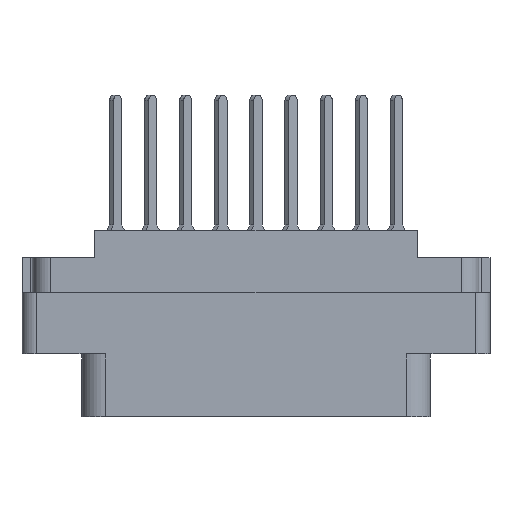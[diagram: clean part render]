
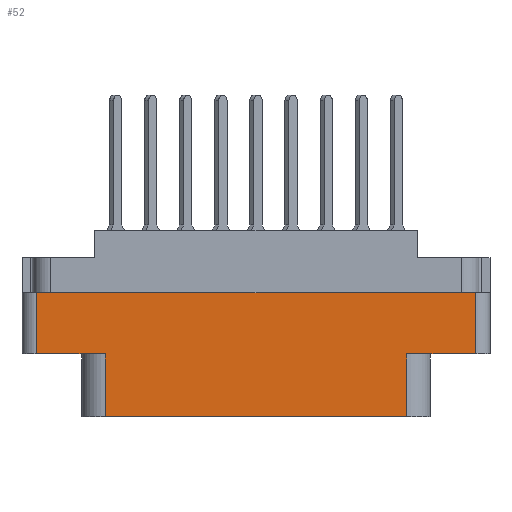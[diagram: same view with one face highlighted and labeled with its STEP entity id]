
A CAD part, front view. The second image highlights one B-rep face of the part: STEP entity #52.
In plain terms, the highlighted planar face has unit normal (0, -1, 0).
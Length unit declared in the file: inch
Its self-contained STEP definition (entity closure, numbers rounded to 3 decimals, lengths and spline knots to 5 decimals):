
#52 = ADVANCED_FACE ( 'NONE', ( #8722 ), #30549, .T. ) ;
#787 = DIRECTION ( 'NONE',  ( 1., 0., 0. ) ) ;
#976 = CARTESIAN_POINT ( 'NONE',  ( 0.644, -0.438, -0.798 ) ) ;
#1190 = DIRECTION ( 'NONE',  ( 1., 0., 0. ) ) ;
#1614 = LINE ( 'NONE', #27000, #14510 ) ;
#1641 = VERTEX_POINT ( 'NONE', #27500 ) ;
#3336 = ORIENTED_EDGE ( 'NONE', *, *, #4127, .F. ) ;
#4081 = CARTESIAN_POINT ( 'NONE',  ( -0.938, -0.438, -0.798 ) ) ;
#4127 = EDGE_CURVE ( 'NONE', #13085, #1641, #29717, .T. ) ;
#4637 = VERTEX_POINT ( 'NONE', #976 ) ;
#5229 = CARTESIAN_POINT ( 'NONE',  ( -1., -0.438, -0.268 ) ) ;
#5317 = EDGE_CURVE ( 'NONE', #13085, #31289, #1614, .T. ) ;
#5384 = DIRECTION ( 'NONE',  ( -1., 0., 0. ) ) ;
#5725 = DIRECTION ( 'NONE',  ( 0., -1., 0. ) ) ;
#6505 = VERTEX_POINT ( 'NONE', #16839 ) ;
#7265 = LINE ( 'NONE', #11999, #16705 ) ;
#7801 = EDGE_LOOP ( 'NONE', ( #8703, #9466, #13724, #3336, #32241, #9646, #20688, #8863 ) ) ;
#7983 = DIRECTION ( 'NONE',  ( 0., 0., -1. ) ) ;
#8046 = DIRECTION ( 'NONE',  ( 1., 0., 0. ) ) ;
#8423 = CARTESIAN_POINT ( 'NONE',  ( -0.938, -0.438, -0.268 ) ) ;
#8432 = CARTESIAN_POINT ( 'NONE',  ( 0., -0.438, -0.529 ) ) ;
#8542 = EDGE_CURVE ( 'NONE', #1641, #4637, #7265, .T. ) ;
#8703 = ORIENTED_EDGE ( 'NONE', *, *, #16300, .T. ) ;
#8722 = FACE_OUTER_BOUND ( 'NONE', #7801, .T. ) ;
#8863 = ORIENTED_EDGE ( 'NONE', *, *, #18747, .T. ) ;
#8896 = CARTESIAN_POINT ( 'NONE',  ( -0.938, -0.438, -0.529 ) ) ;
#9466 = ORIENTED_EDGE ( 'NONE', *, *, #31566, .T. ) ;
#9646 = ORIENTED_EDGE ( 'NONE', *, *, #26502, .F. ) ;
#10174 = LINE ( 'NONE', #5229, #15712 ) ;
#10607 = VERTEX_POINT ( 'NONE', #23777 ) ;
#11999 = CARTESIAN_POINT ( 'NONE',  ( 0.644, -0.438, -0.529 ) ) ;
#12372 = DIRECTION ( 'NONE',  ( 0., 0., 1. ) ) ;
#12681 = CARTESIAN_POINT ( 'NONE',  ( 0.938, -0.438, -0.268 ) ) ;
#13085 = VERTEX_POINT ( 'NONE', #28790 ) ;
#13250 = AXIS2_PLACEMENT_3D ( 'NONE', #13253, #5725, #7983 ) ;
#13253 = CARTESIAN_POINT ( 'NONE',  ( -0.938, -0.438, -0.798 ) ) ;
#13724 = ORIENTED_EDGE ( 'NONE', *, *, #8542, .F. ) ;
#14510 = VECTOR ( 'NONE', #17215, 39.37008 ) ;
#14715 = VECTOR ( 'NONE', #787, 39.37008 ) ;
#15229 = DIRECTION ( 'NONE',  ( 0., 0., -1. ) ) ;
#15712 = VECTOR ( 'NONE', #8046, 39.37008 ) ;
#16188 = EDGE_CURVE ( 'NONE', #23786, #16444, #28349, .T. ) ;
#16300 = EDGE_CURVE ( 'NONE', #6505, #10607, #24042, .T. ) ;
#16444 = VERTEX_POINT ( 'NONE', #8423 ) ;
#16563 = DIRECTION ( 'NONE',  ( 0., 0., -1. ) ) ;
#16705 = VECTOR ( 'NONE', #16563, 39.37008 ) ;
#16839 = CARTESIAN_POINT ( 'NONE',  ( -0.644, -0.438, -0.529 ) ) ;
#17092 = VECTOR ( 'NONE', #1190, 39.37008 ) ;
#17215 = DIRECTION ( 'NONE',  ( 0., 0., 1. ) ) ;
#18747 = EDGE_CURVE ( 'NONE', #23786, #6505, #19066, .T. ) ;
#19066 = LINE ( 'NONE', #8432, #14715 ) ;
#19281 = VECTOR ( 'NONE', #15229, 39.37008 ) ;
#20405 = CARTESIAN_POINT ( 'NONE',  ( 0., -0.438, -0.529 ) ) ;
#20688 = ORIENTED_EDGE ( 'NONE', *, *, #16188, .F. ) ;
#22978 = LINE ( 'NONE', #4081, #17092 ) ;
#23049 = CARTESIAN_POINT ( 'NONE',  ( -0.644, -0.438, -0.529 ) ) ;
#23777 = CARTESIAN_POINT ( 'NONE',  ( -0.644, -0.438, -0.798 ) ) ;
#23786 = VERTEX_POINT ( 'NONE', #8896 ) ;
#24042 = LINE ( 'NONE', #23049, #19281 ) ;
#26502 = EDGE_CURVE ( 'NONE', #16444, #31289, #10174, .T. ) ;
#27000 = CARTESIAN_POINT ( 'NONE',  ( 0.938, -0.438, -0.798 ) ) ;
#27500 = CARTESIAN_POINT ( 'NONE',  ( 0.644, -0.438, -0.529 ) ) ;
#28349 = LINE ( 'NONE', #29770, #31889 ) ;
#28790 = CARTESIAN_POINT ( 'NONE',  ( 0.938, -0.438, -0.529 ) ) ;
#29717 = LINE ( 'NONE', #20405, #32482 ) ;
#29770 = CARTESIAN_POINT ( 'NONE',  ( -0.938, -0.438, -0.798 ) ) ;
#30549 = PLANE ( 'NONE',  #13250 ) ;
#31289 = VERTEX_POINT ( 'NONE', #12681 ) ;
#31566 = EDGE_CURVE ( 'NONE', #10607, #4637, #22978, .T. ) ;
#31889 = VECTOR ( 'NONE', #12372, 39.37008 ) ;
#32241 = ORIENTED_EDGE ( 'NONE', *, *, #5317, .T. ) ;
#32482 = VECTOR ( 'NONE', #5384, 39.37008 ) ;
